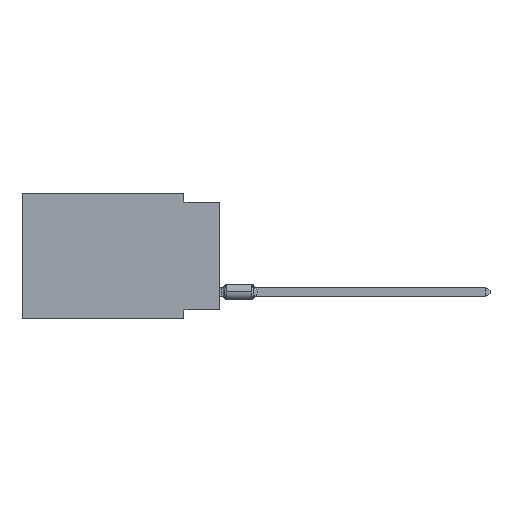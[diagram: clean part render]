
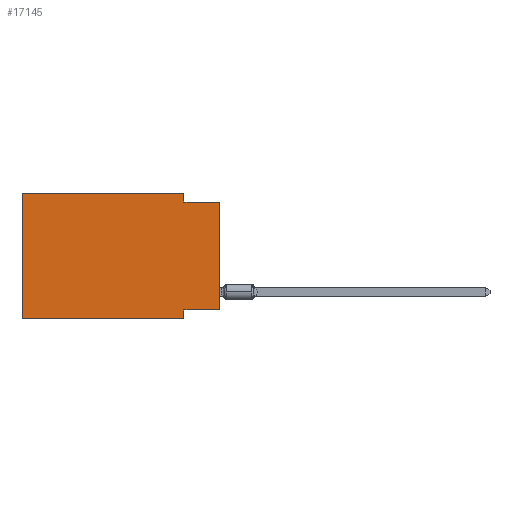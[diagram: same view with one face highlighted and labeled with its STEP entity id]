
A CAD part, left-side view. The second image highlights one B-rep face of the part: STEP entity #17145.
In plain terms, the highlighted planar face has unit normal (-1, 0, 0).
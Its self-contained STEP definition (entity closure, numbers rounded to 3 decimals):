
#347 = LINE ( 'NONE', #11460, #28833 ) ;
#426 = DIRECTION ( 'NONE',  ( 0., -1., 0. ) ) ;
#2198 = LINE ( 'NONE', #10396, #14432 ) ;
#2408 = ORIENTED_EDGE ( 'NONE', *, *, #2583, .F. ) ;
#2583 = EDGE_CURVE ( 'NONE', #20396, #18892, #12447, .T. ) ;
#2727 = ORIENTED_EDGE ( 'NONE', *, *, #13710, .F. ) ;
#3327 = CARTESIAN_POINT ( 'NONE',  ( 0., 13.97, 0. ) ) ;
#3916 = CARTESIAN_POINT ( 'NONE',  ( 0., 2.54, 0. ) ) ;
#4193 = EDGE_CURVE ( 'NONE', #20358, #26512, #23632, .T. ) ;
#4260 = VECTOR ( 'NONE', #26888, 1000. ) ;
#4388 = CARTESIAN_POINT ( 'NONE',  ( 0., 2.54, 0. ) ) ;
#4539 = DIRECTION ( 'NONE',  ( 0., 0., -1. ) ) ;
#5645 = EDGE_CURVE ( 'NONE', #12457, #12309, #31241, .T. ) ;
#5730 = VECTOR ( 'NONE', #14665, 1000. ) ;
#6071 = CARTESIAN_POINT ( 'NONE',  ( 0., 13.97, 0. ) ) ;
#6545 = VECTOR ( 'NONE', #426, 1000. ) ;
#6783 = CARTESIAN_POINT ( 'NONE',  ( 0., 2.54, -8.255 ) ) ;
#7400 = CARTESIAN_POINT ( 'NONE',  ( 0., 0., 0. ) ) ;
#8565 = DIRECTION ( 'NONE',  ( 0., 1., 0. ) ) ;
#8804 = CARTESIAN_POINT ( 'NONE',  ( 0., 0., -0.635 ) ) ;
#8878 = DIRECTION ( 'NONE',  ( 0., -1., 0. ) ) ;
#8975 = VERTEX_POINT ( 'NONE', #34620 ) ;
#9106 = ORIENTED_EDGE ( 'NONE', *, *, #4193, .T. ) ;
#9323 = DIRECTION ( 'NONE',  ( 0., 0., 1. ) ) ;
#10396 = CARTESIAN_POINT ( 'NONE',  ( 0., 2.54, -8.89 ) ) ;
#11460 = CARTESIAN_POINT ( 'NONE',  ( 0., 0., -0.635 ) ) ;
#11686 = CARTESIAN_POINT ( 'NONE',  ( 0., 2.54, -0.635 ) ) ;
#12309 = VERTEX_POINT ( 'NONE', #11686 ) ;
#12447 = LINE ( 'NONE', #6071, #20489 ) ;
#12457 = VERTEX_POINT ( 'NONE', #4388 ) ;
#13244 = DIRECTION ( 'NONE',  ( 0., 0., 1. ) ) ;
#13710 = EDGE_CURVE ( 'NONE', #23859, #8975, #2198, .T. ) ;
#14432 = VECTOR ( 'NONE', #19133, 1000. ) ;
#14665 = DIRECTION ( 'NONE',  ( 0., 0., -1. ) ) ;
#15654 = FACE_OUTER_BOUND ( 'NONE', #18318, .T. ) ;
#16117 = ORIENTED_EDGE ( 'NONE', *, *, #17717, .F. ) ;
#17145 = ADVANCED_FACE ( 'NONE', ( #15654 ), #32930, .F. ) ;
#17717 = EDGE_CURVE ( 'NONE', #18892, #12457, #25375, .T. ) ;
#18318 = EDGE_LOOP ( 'NONE', ( #9106, #25553, #35464, #16117, #2408, #22920, #2727, #23275 ) ) ;
#18892 = VERTEX_POINT ( 'NONE', #28329 ) ;
#19133 = DIRECTION ( 'NONE',  ( 0., 0., -1. ) ) ;
#20358 = VERTEX_POINT ( 'NONE', #23835 ) ;
#20396 = VERTEX_POINT ( 'NONE', #33471 ) ;
#20489 = VECTOR ( 'NONE', #9323, 1000. ) ;
#21634 = CARTESIAN_POINT ( 'NONE',  ( 0., 13.97, 0. ) ) ;
#22762 = LINE ( 'NONE', #24789, #30425 ) ;
#22920 = ORIENTED_EDGE ( 'NONE', *, *, #34948, .T. ) ;
#23275 = ORIENTED_EDGE ( 'NONE', *, *, #34210, .F. ) ;
#23632 = LINE ( 'NONE', #7400, #32063 ) ;
#23835 = CARTESIAN_POINT ( 'NONE',  ( 0., 0., -8.255 ) ) ;
#23859 = VERTEX_POINT ( 'NONE', #6783 ) ;
#24552 = DIRECTION ( 'NONE',  ( 1., 0., 0. ) ) ;
#24789 = CARTESIAN_POINT ( 'NONE',  ( 0., 0., -8.255 ) ) ;
#25375 = LINE ( 'NONE', #3327, #6545 ) ;
#25553 = ORIENTED_EDGE ( 'NONE', *, *, #30777, .F. ) ;
#26355 = LINE ( 'NONE', #29796, #4260 ) ;
#26512 = VERTEX_POINT ( 'NONE', #8804 ) ;
#26888 = DIRECTION ( 'NONE',  ( 0., -1., 0. ) ) ;
#28329 = CARTESIAN_POINT ( 'NONE',  ( 0., 13.97, 0. ) ) ;
#28833 = VECTOR ( 'NONE', #8878, 1000. ) ;
#29796 = CARTESIAN_POINT ( 'NONE',  ( 0., 13.97, -8.89 ) ) ;
#30425 = VECTOR ( 'NONE', #8565, 1000. ) ;
#30777 = EDGE_CURVE ( 'NONE', #12309, #26512, #347, .T. ) ;
#31241 = LINE ( 'NONE', #3916, #5730 ) ;
#32063 = VECTOR ( 'NONE', #13244, 1000. ) ;
#32930 = PLANE ( 'NONE',  #35027 ) ;
#33471 = CARTESIAN_POINT ( 'NONE',  ( 0., 13.97, -8.89 ) ) ;
#34210 = EDGE_CURVE ( 'NONE', #20358, #23859, #22762, .T. ) ;
#34620 = CARTESIAN_POINT ( 'NONE',  ( 0., 2.54, -8.89 ) ) ;
#34948 = EDGE_CURVE ( 'NONE', #20396, #8975, #26355, .T. ) ;
#35027 = AXIS2_PLACEMENT_3D ( 'NONE', #21634, #24552, #4539 ) ;
#35464 = ORIENTED_EDGE ( 'NONE', *, *, #5645, .F. ) ;
